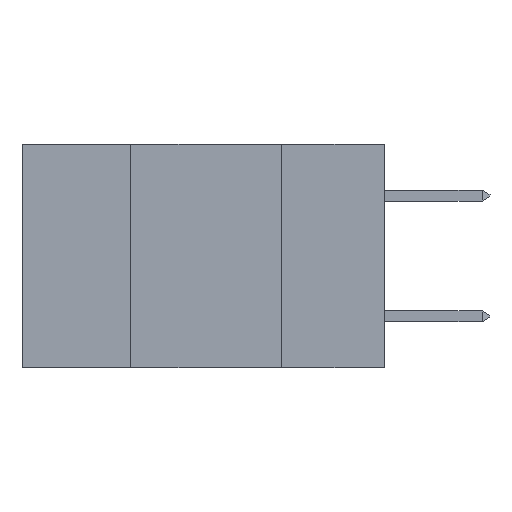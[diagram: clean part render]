
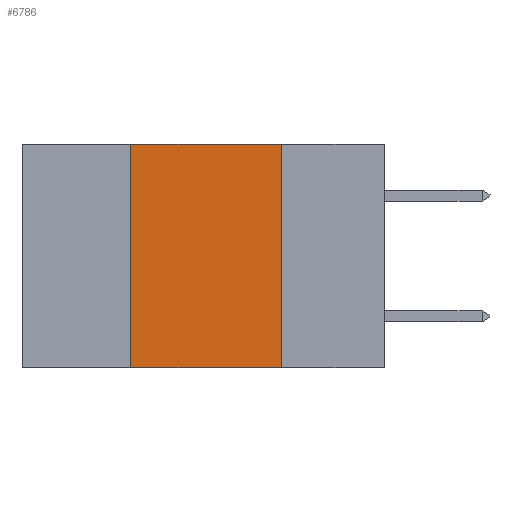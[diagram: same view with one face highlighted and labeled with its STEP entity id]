
A CAD part, left-side view. The second image highlights one B-rep face of the part: STEP entity #6786.
In plain terms, the highlighted planar face has unit normal (-1, 0, 0).
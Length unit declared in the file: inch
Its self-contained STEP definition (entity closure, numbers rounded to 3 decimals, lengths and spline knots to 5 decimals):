
#772 = CARTESIAN_POINT ( 'NONE',  ( 0., 0.42, -0.37 ) ) ;
#906 = ORIENTED_EDGE ( 'NONE', *, *, #18744, .F. ) ;
#2090 = EDGE_CURVE ( 'NONE', #14436, #20441, #6232, .T. ) ;
#2286 = VECTOR ( 'NONE', #17022, 39.37008 ) ;
#2741 = EDGE_LOOP ( 'NONE', ( #906, #12412, #3904, #4645 ) ) ;
#3904 = ORIENTED_EDGE ( 'NONE', *, *, #2090, .F. ) ;
#3941 = VECTOR ( 'NONE', #18415, 39.37008 ) ;
#4377 = VECTOR ( 'NONE', #10255, 39.37008 ) ;
#4645 = ORIENTED_EDGE ( 'NONE', *, *, #14507, .T. ) ;
#4900 = LINE ( 'NONE', #6878, #4377 ) ;
#5132 = CARTESIAN_POINT ( 'NONE',  ( 0., 0.17, 0. ) ) ;
#6232 = LINE ( 'NONE', #17001, #2286 ) ;
#6786 = ADVANCED_FACE ( 'NONE', ( #7175 ), #10875, .F. ) ;
#6878 = CARTESIAN_POINT ( 'NONE',  ( 0., 0.6, 0. ) ) ;
#7021 = LINE ( 'NONE', #9337, #10948 ) ;
#7175 = FACE_OUTER_BOUND ( 'NONE', #2741, .T. ) ;
#7583 = CARTESIAN_POINT ( 'NONE',  ( 0., 0.6, 0. ) ) ;
#8483 = VERTEX_POINT ( 'NONE', #11672 ) ;
#9217 = AXIS2_PLACEMENT_3D ( 'NONE', #7583, #19101, #9271 ) ;
#9271 = DIRECTION ( 'NONE',  ( 0., 0., -1. ) ) ;
#9337 = CARTESIAN_POINT ( 'NONE',  ( 0., 0.6, -0.37 ) ) ;
#10255 = DIRECTION ( 'NONE',  ( 0., -1., 0. ) ) ;
#10875 = PLANE ( 'NONE',  #9217 ) ;
#10948 = VECTOR ( 'NONE', #17618, 39.37008 ) ;
#11672 = CARTESIAN_POINT ( 'NONE',  ( 0., 0.17, 0. ) ) ;
#12139 = VERTEX_POINT ( 'NONE', #21472 ) ;
#12366 = LINE ( 'NONE', #5132, #3941 ) ;
#12412 = ORIENTED_EDGE ( 'NONE', *, *, #13490, .F. ) ;
#13490 = EDGE_CURVE ( 'NONE', #20441, #8483, #4900, .T. ) ;
#14436 = VERTEX_POINT ( 'NONE', #772 ) ;
#14507 = EDGE_CURVE ( 'NONE', #14436, #12139, #7021, .T. ) ;
#17001 = CARTESIAN_POINT ( 'NONE',  ( 0., 0.42, 0. ) ) ;
#17022 = DIRECTION ( 'NONE',  ( 0., 0., 1. ) ) ;
#17618 = DIRECTION ( 'NONE',  ( 0., -1., 0. ) ) ;
#18415 = DIRECTION ( 'NONE',  ( 0., 0., -1. ) ) ;
#18744 = EDGE_CURVE ( 'NONE', #8483, #12139, #12366, .T. ) ;
#19101 = DIRECTION ( 'NONE',  ( 1., 0., 0. ) ) ;
#19189 = CARTESIAN_POINT ( 'NONE',  ( 0., 0.42, 0. ) ) ;
#20441 = VERTEX_POINT ( 'NONE', #19189 ) ;
#21472 = CARTESIAN_POINT ( 'NONE',  ( 0., 0.17, -0.37 ) ) ;
